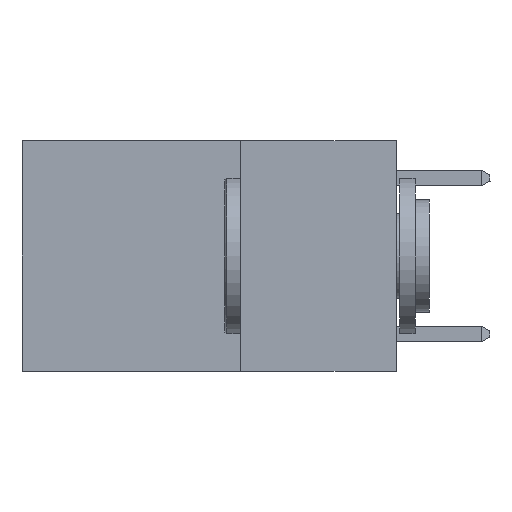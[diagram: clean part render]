
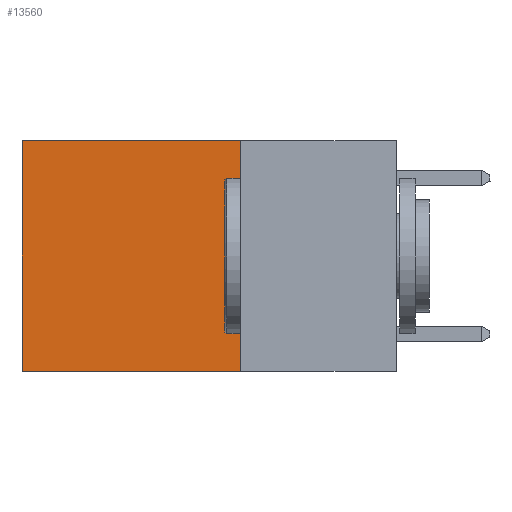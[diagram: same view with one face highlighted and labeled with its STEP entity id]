
A CAD part, left-side view. The second image highlights one B-rep face of the part: STEP entity #13560.
In plain terms, the highlighted planar face has unit normal (-1, 0, 0).
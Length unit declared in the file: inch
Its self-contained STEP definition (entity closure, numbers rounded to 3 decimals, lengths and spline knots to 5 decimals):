
#108 = EDGE_CURVE ( 'NONE', #12693, #10932, #11710, .T. ) ;
#670 = VERTEX_POINT ( 'NONE', #5754 ) ;
#1308 = CARTESIAN_POINT ( 'NONE',  ( 0.2625, 0.6, -0.37 ) ) ;
#1740 = VECTOR ( 'NONE', #6105, 39.37008 ) ;
#1774 = CARTESIAN_POINT ( 'NONE',  ( 0.2625, 0.25, 0. ) ) ;
#1845 = DIRECTION ( 'NONE',  ( 0., 0., -1. ) ) ;
#2177 = LINE ( 'NONE', #4933, #12719 ) ;
#3436 = CARTESIAN_POINT ( 'NONE',  ( 0.2625, 0.25, 0. ) ) ;
#3803 = ORIENTED_EDGE ( 'NONE', *, *, #7848, .F. ) ;
#4420 = DIRECTION ( 'NONE',  ( 0., 0., -1. ) ) ;
#4878 = DIRECTION ( 'NONE',  ( 1., 0., 0. ) ) ;
#4933 = CARTESIAN_POINT ( 'NONE',  ( 0.2625, 0.6, 0. ) ) ;
#5525 = LINE ( 'NONE', #3436, #12565 ) ;
#5754 = CARTESIAN_POINT ( 'NONE',  ( 0.2625, 0.25, -0.37 ) ) ;
#5765 = VECTOR ( 'NONE', #8951, 39.37008 ) ;
#6105 = DIRECTION ( 'NONE',  ( 0., 1., 0. ) ) ;
#6787 = EDGE_LOOP ( 'NONE', ( #8239, #3803, #10310, #10476 ) ) ;
#7288 = PLANE ( 'NONE',  #8997 ) ;
#7306 = CARTESIAN_POINT ( 'NONE',  ( 0.2625, 0.25, 0. ) ) ;
#7468 = CARTESIAN_POINT ( 'NONE',  ( 0.2625, 0.25, 0. ) ) ;
#7479 = EDGE_CURVE ( 'NONE', #10932, #13098, #2177, .T. ) ;
#7848 = EDGE_CURVE ( 'NONE', #670, #13098, #11059, .T. ) ;
#8239 = ORIENTED_EDGE ( 'NONE', *, *, #7479, .T. ) ;
#8814 = CARTESIAN_POINT ( 'NONE',  ( 0.2625, 0.25, -0.37 ) ) ;
#8951 = DIRECTION ( 'NONE',  ( 0., 1., 0. ) ) ;
#8997 = AXIS2_PLACEMENT_3D ( 'NONE', #1774, #4878, #1845 ) ;
#10310 = ORIENTED_EDGE ( 'NONE', *, *, #11577, .F. ) ;
#10476 = ORIENTED_EDGE ( 'NONE', *, *, #108, .T. ) ;
#10932 = VERTEX_POINT ( 'NONE', #11161 ) ;
#11059 = LINE ( 'NONE', #8814, #5765 ) ;
#11161 = CARTESIAN_POINT ( 'NONE',  ( 0.2625, 0.6, 0. ) ) ;
#11577 = EDGE_CURVE ( 'NONE', #12693, #670, #5525, .T. ) ;
#11710 = LINE ( 'NONE', #7468, #1740 ) ;
#12565 = VECTOR ( 'NONE', #4420, 39.37008 ) ;
#12693 = VERTEX_POINT ( 'NONE', #7306 ) ;
#12719 = VECTOR ( 'NONE', #13638, 39.37008 ) ;
#13098 = VERTEX_POINT ( 'NONE', #1308 ) ;
#13560 = ADVANCED_FACE ( 'NONE', ( #13708 ), #7288, .F. ) ;
#13638 = DIRECTION ( 'NONE',  ( 0., 0., -1. ) ) ;
#13708 = FACE_OUTER_BOUND ( 'NONE', #6787, .T. ) ;
